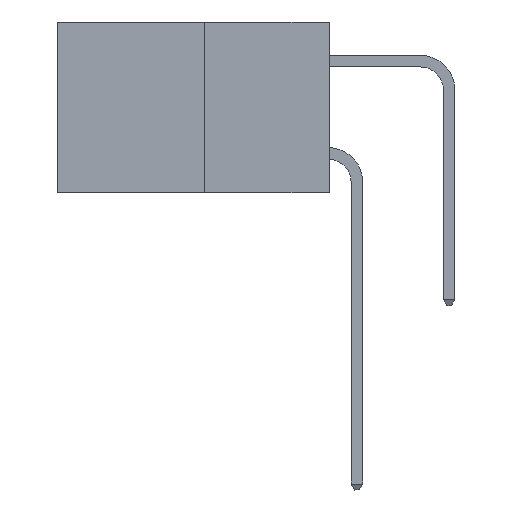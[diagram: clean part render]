
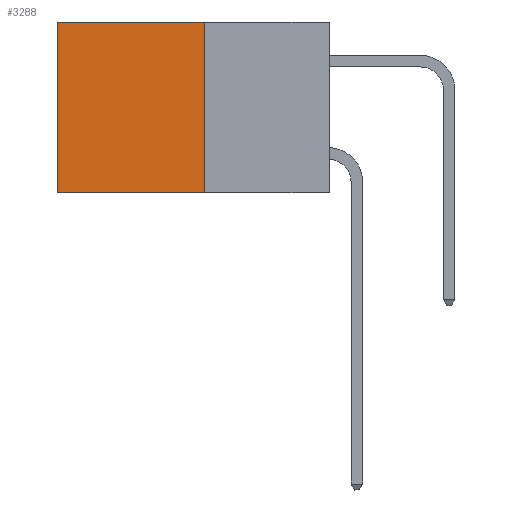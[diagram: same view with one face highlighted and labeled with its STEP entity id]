
A CAD part, left-side view. The second image highlights one B-rep face of the part: STEP entity #3288.
In plain terms, the highlighted planar face has unit normal (-1, 0, 0).
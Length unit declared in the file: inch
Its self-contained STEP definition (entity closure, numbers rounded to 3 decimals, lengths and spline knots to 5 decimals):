
#243 = PLANE ( 'NONE',  #10693 ) ;
#1744 = CARTESIAN_POINT ( 'NONE',  ( 0.277, 0.27, -0.37 ) ) ;
#2017 = ORIENTED_EDGE ( 'NONE', *, *, #17996, .T. ) ;
#2046 = CARTESIAN_POINT ( 'NONE',  ( 0.277, 0.59, 0. ) ) ;
#3288 = ADVANCED_FACE ( 'NONE', ( #19776 ), #243, .F. ) ;
#3339 = VERTEX_POINT ( 'NONE', #5721 ) ;
#3449 = VECTOR ( 'NONE', #11685, 39.37008 ) ;
#3719 = ORIENTED_EDGE ( 'NONE', *, *, #20173, .F. ) ;
#3934 = ORIENTED_EDGE ( 'NONE', *, *, #7150, .F. ) ;
#5721 = CARTESIAN_POINT ( 'NONE',  ( 0.277, 0.59, -0.37 ) ) ;
#5931 = CARTESIAN_POINT ( 'NONE',  ( 0.277, 0.59, -0.37 ) ) ;
#6002 = DIRECTION ( 'NONE',  ( 1., 0., 0. ) ) ;
#6270 = CARTESIAN_POINT ( 'NONE',  ( 0.277, 0.27, -0.37 ) ) ;
#7094 = VECTOR ( 'NONE', #20213, 39.37008 ) ;
#7150 = EDGE_CURVE ( 'NONE', #16765, #3339, #11874, .T. ) ;
#7682 = VECTOR ( 'NONE', #20093, 39.37008 ) ;
#7785 = EDGE_LOOP ( 'NONE', ( #2017, #3934, #3719, #18158 ) ) ;
#8161 = VERTEX_POINT ( 'NONE', #2046 ) ;
#9234 = DIRECTION ( 'NONE',  ( 0., 0., -1. ) ) ;
#9735 = LINE ( 'NONE', #5931, #18204 ) ;
#10693 = AXIS2_PLACEMENT_3D ( 'NONE', #20113, #6002, #9234 ) ;
#11685 = DIRECTION ( 'NONE',  ( 0., 0., -1. ) ) ;
#11874 = LINE ( 'NONE', #20126, #7094 ) ;
#12148 = LINE ( 'NONE', #1744, #3449 ) ;
#13762 = CARTESIAN_POINT ( 'NONE',  ( 0.277, 0.27, 0. ) ) ;
#15508 = DIRECTION ( 'NONE',  ( 0., 0., -1. ) ) ;
#16415 = CARTESIAN_POINT ( 'NONE',  ( 0.277, 0.27, 0. ) ) ;
#16765 = VERTEX_POINT ( 'NONE', #6270 ) ;
#17996 = EDGE_CURVE ( 'NONE', #8161, #3339, #9735, .T. ) ;
#18158 = ORIENTED_EDGE ( 'NONE', *, *, #18809, .T. ) ;
#18204 = VECTOR ( 'NONE', #15508, 39.37008 ) ;
#18809 = EDGE_CURVE ( 'NONE', #19379, #8161, #20353, .T. ) ;
#19379 = VERTEX_POINT ( 'NONE', #16415 ) ;
#19776 = FACE_OUTER_BOUND ( 'NONE', #7785, .T. ) ;
#20093 = DIRECTION ( 'NONE',  ( 0., 1., 0. ) ) ;
#20113 = CARTESIAN_POINT ( 'NONE',  ( 0.277, 0.27, -0.37 ) ) ;
#20126 = CARTESIAN_POINT ( 'NONE',  ( 0.277, 0.27, -0.37 ) ) ;
#20173 = EDGE_CURVE ( 'NONE', #19379, #16765, #12148, .T. ) ;
#20213 = DIRECTION ( 'NONE',  ( 0., 1., 0. ) ) ;
#20353 = LINE ( 'NONE', #13762, #7682 ) ;
